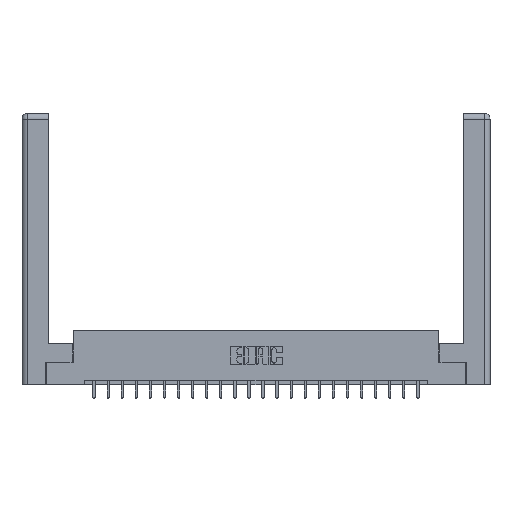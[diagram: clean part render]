
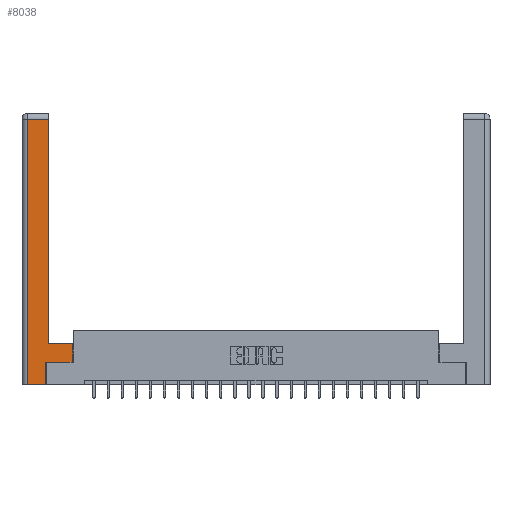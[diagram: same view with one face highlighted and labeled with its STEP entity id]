
A CAD part, top view. The second image highlights one B-rep face of the part: STEP entity #8038.
In plain terms, the highlighted planar face has unit normal (0, 0, 1).
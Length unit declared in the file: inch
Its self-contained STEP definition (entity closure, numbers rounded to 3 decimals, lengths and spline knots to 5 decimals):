
#46 = ORIENTED_EDGE ( 'NONE', *, *, #468, .T. ) ;
#127 = VECTOR ( 'NONE', #3057, 39.37008 ) ;
#468 = EDGE_CURVE ( 'NONE', #9180, #16942, #21533, .T. ) ;
#641 = VECTOR ( 'NONE', #9175, 39.37008 ) ;
#646 = CARTESIAN_POINT ( 'NONE',  ( 0.295, 0.45, 0. ) ) ;
#1224 = CARTESIAN_POINT ( 'NONE',  ( 0.295, 3., 0. ) ) ;
#1332 = CARTESIAN_POINT ( 'NONE',  ( 0.0615, 0., 0. ) ) ;
#1383 = DIRECTION ( 'NONE',  ( 0., -1., 0. ) ) ;
#1819 = VECTOR ( 'NONE', #10703, 39.37008 ) ;
#2226 = LINE ( 'NONE', #14400, #16201 ) ;
#2367 = LINE ( 'NONE', #20786, #14612 ) ;
#2773 = ORIENTED_EDGE ( 'NONE', *, *, #8979, .T. ) ;
#3057 = DIRECTION ( 'NONE',  ( 0., 1., 0. ) ) ;
#3087 = LINE ( 'NONE', #12784, #18759 ) ;
#3467 = ORIENTED_EDGE ( 'NONE', *, *, #4799, .T. ) ;
#4209 = CARTESIAN_POINT ( 'NONE',  ( 0.565, 0.45, 0. ) ) ;
#4799 = EDGE_CURVE ( 'NONE', #16532, #20074, #6584, .T. ) ;
#5979 = ORIENTED_EDGE ( 'NONE', *, *, #12480, .T. ) ;
#6169 = FACE_OUTER_BOUND ( 'NONE', #13740, .T. ) ;
#6409 = EDGE_CURVE ( 'NONE', #19838, #16532, #3087, .T. ) ;
#6443 = LINE ( 'NONE', #14313, #1819 ) ;
#6584 = LINE ( 'NONE', #8688, #15083 ) ;
#6688 = EDGE_CURVE ( 'NONE', #13969, #21827, #2226, .T. ) ;
#7252 = DIRECTION ( 'NONE',  ( -1., 0., 0. ) ) ;
#7988 = EDGE_CURVE ( 'NONE', #20074, #9180, #6443, .T. ) ;
#8038 = ADVANCED_FACE ( 'NONE', ( #6169 ), #9004, .F. ) ;
#8688 = CARTESIAN_POINT ( 'NONE',  ( 0.0615, 0., 0. ) ) ;
#8979 = EDGE_CURVE ( 'NONE', #16942, #13969, #13469, .T. ) ;
#9004 = PLANE ( 'NONE',  #9404 ) ;
#9147 = EDGE_CURVE ( 'NONE', #21827, #10871, #2367, .T. ) ;
#9175 = DIRECTION ( 'NONE',  ( 1., 0., 0. ) ) ;
#9180 = VERTEX_POINT ( 'NONE', #21322 ) ;
#9326 = DIRECTION ( 'NONE',  ( -1., 0., 0. ) ) ;
#9342 = CARTESIAN_POINT ( 'NONE',  ( 0.0615, 2.94, 0. ) ) ;
#9404 = AXIS2_PLACEMENT_3D ( 'NONE', #16320, #18143, #7252 ) ;
#9862 = DIRECTION ( 'NONE',  ( -1., 0., 0. ) ) ;
#10637 = DIRECTION ( 'NONE',  ( 0., 1., 0. ) ) ;
#10703 = DIRECTION ( 'NONE',  ( 1., 0., 0. ) ) ;
#10846 = VECTOR ( 'NONE', #12054, 39.37008 ) ;
#10871 = VERTEX_POINT ( 'NONE', #646 ) ;
#12054 = DIRECTION ( 'NONE',  ( 0., 1., 0. ) ) ;
#12308 = ORIENTED_EDGE ( 'NONE', *, *, #6409, .T. ) ;
#12480 = EDGE_CURVE ( 'NONE', #10871, #19838, #21172, .T. ) ;
#12784 = CARTESIAN_POINT ( 'NONE',  ( 0.0615, 2.94, 0. ) ) ;
#13469 = LINE ( 'NONE', #19832, #641 ) ;
#13740 = EDGE_LOOP ( 'NONE', ( #5979, #12308, #3467, #17953, #46, #2773, #16102, #20415 ) ) ;
#13969 = VERTEX_POINT ( 'NONE', #23538 ) ;
#14313 = CARTESIAN_POINT ( 'NONE',  ( 0.265, 0., 0. ) ) ;
#14400 = CARTESIAN_POINT ( 'NONE',  ( 0.565, 0.45, 0. ) ) ;
#14612 = VECTOR ( 'NONE', #9862, 39.37008 ) ;
#15083 = VECTOR ( 'NONE', #1383, 39.37008 ) ;
#15632 = CARTESIAN_POINT ( 'NONE',  ( 0.265, 0.245, 0. ) ) ;
#16102 = ORIENTED_EDGE ( 'NONE', *, *, #6688, .T. ) ;
#16201 = VECTOR ( 'NONE', #10637, 39.37008 ) ;
#16320 = CARTESIAN_POINT ( 'NONE',  ( 0., 0., 0. ) ) ;
#16532 = VERTEX_POINT ( 'NONE', #9342 ) ;
#16942 = VERTEX_POINT ( 'NONE', #20474 ) ;
#17953 = ORIENTED_EDGE ( 'NONE', *, *, #7988, .T. ) ;
#18143 = DIRECTION ( 'NONE',  ( 0., 0., -1. ) ) ;
#18759 = VECTOR ( 'NONE', #9326, 39.37008 ) ;
#19832 = CARTESIAN_POINT ( 'NONE',  ( 0.565, 0.245, 0. ) ) ;
#19838 = VERTEX_POINT ( 'NONE', #22086 ) ;
#20074 = VERTEX_POINT ( 'NONE', #1332 ) ;
#20415 = ORIENTED_EDGE ( 'NONE', *, *, #9147, .T. ) ;
#20474 = CARTESIAN_POINT ( 'NONE',  ( 0.265, 0.245, 0. ) ) ;
#20786 = CARTESIAN_POINT ( 'NONE',  ( 0.295, 0.45, 0. ) ) ;
#21172 = LINE ( 'NONE', #1224, #10846 ) ;
#21322 = CARTESIAN_POINT ( 'NONE',  ( 0.265, 0., 0. ) ) ;
#21533 = LINE ( 'NONE', #15632, #127 ) ;
#21827 = VERTEX_POINT ( 'NONE', #4209 ) ;
#22086 = CARTESIAN_POINT ( 'NONE',  ( 0.295, 2.94, 0. ) ) ;
#23538 = CARTESIAN_POINT ( 'NONE',  ( 0.565, 0.245, 0. ) ) ;
